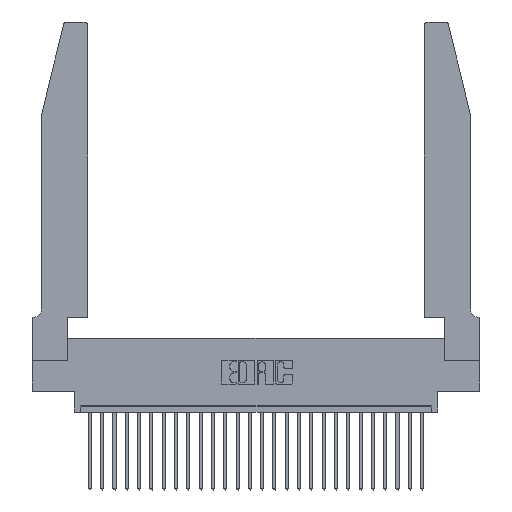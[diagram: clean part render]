
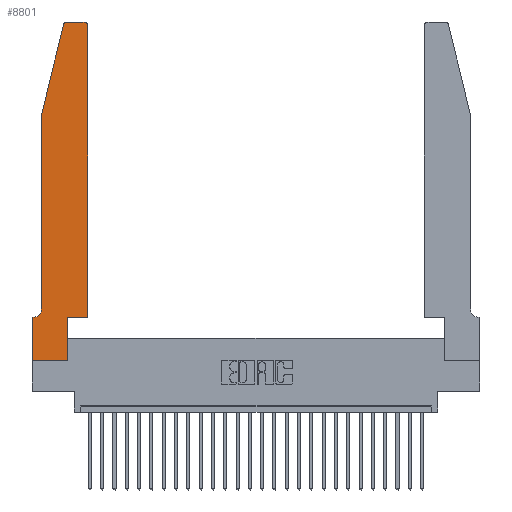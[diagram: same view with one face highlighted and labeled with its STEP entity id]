
A CAD part, top view. The second image highlights one B-rep face of the part: STEP entity #8801.
In plain terms, the highlighted planar face has unit normal (0, 0, 1).
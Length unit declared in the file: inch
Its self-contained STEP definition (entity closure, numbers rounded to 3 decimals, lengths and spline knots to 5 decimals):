
#81 = VERTEX_POINT ( 'NONE', #21621 ) ;
#365 = ORIENTED_EDGE ( 'NONE', *, *, #10234, .T. ) ;
#627 = DIRECTION ( 'NONE',  ( 0., 0., 1. ) ) ;
#1090 = CARTESIAN_POINT ( 'NONE',  ( 0.4205, 2.75, 0.37 ) ) ;
#1099 = EDGE_CURVE ( 'NONE', #7699, #81, #10489, .T. ) ;
#1174 = VECTOR ( 'NONE', #8056, 39.37008 ) ;
#1873 = ORIENTED_EDGE ( 'NONE', *, *, #8863, .T. ) ;
#1979 = DIRECTION ( 'NONE',  ( -0.239, -0.971, 0. ) ) ;
#1986 = CIRCLE ( 'NONE', #18469, 0.03 ) ;
#2052 = CARTESIAN_POINT ( 'NONE',  ( 0., 0., 0.37 ) ) ;
#2058 = CARTESIAN_POINT ( 'NONE',  ( 0.0055, 0.42, 0.37 ) ) ;
#2445 = DIRECTION ( 'NONE',  ( 0., 0., 1. ) ) ;
#2933 = VERTEX_POINT ( 'NONE', #11537 ) ;
#3525 = DIRECTION ( 'NONE',  ( 1., 0., 0. ) ) ;
#3852 = EDGE_CURVE ( 'NONE', #22568, #19547, #4517, .T. ) ;
#3882 = VECTOR ( 'NONE', #3525, 39.37008 ) ;
#4231 = LINE ( 'NONE', #16467, #1174 ) ;
#4517 = LINE ( 'NONE', #2052, #8224 ) ;
#4725 = LINE ( 'NONE', #13788, #12792 ) ;
#5805 = CARTESIAN_POINT ( 'NONE',  ( 0., 0.35, 0.37 ) ) ;
#6285 = EDGE_CURVE ( 'NONE', #2933, #8730, #16114, .T. ) ;
#6507 = DIRECTION ( 'NONE',  ( 0., 1., 0. ) ) ;
#6739 = CARTESIAN_POINT ( 'NONE',  ( 0.2865, 0.35, 0.37 ) ) ;
#7037 = ORIENTED_EDGE ( 'NONE', *, *, #1099, .T. ) ;
#7048 = CARTESIAN_POINT ( 'NONE',  ( 0.25487, 2.72718, 0.37 ) ) ;
#7078 = ORIENTED_EDGE ( 'NONE', *, *, #12783, .T. ) ;
#7085 = VERTEX_POINT ( 'NONE', #16417 ) ;
#7314 = EDGE_CURVE ( 'NONE', #25011, #2933, #10383, .T. ) ;
#7699 = VERTEX_POINT ( 'NONE', #15343 ) ;
#8056 = DIRECTION ( 'NONE',  ( 0., -1., 0. ) ) ;
#8224 = VECTOR ( 'NONE', #12958, 39.37008 ) ;
#8242 = DIRECTION ( 'NONE',  ( 0., 1., 0. ) ) ;
#8587 = PLANE ( 'NONE',  #19742 ) ;
#8730 = VERTEX_POINT ( 'NONE', #18308 ) ;
#8801 = ADVANCED_FACE ( 'NONE', ( #24024 ), #8587, .T. ) ;
#8846 = CARTESIAN_POINT ( 'NONE',  ( 0.4205, 2.72, 0.37 ) ) ;
#8863 = EDGE_CURVE ( 'NONE', #19478, #7699, #4231, .T. ) ;
#8915 = ORIENTED_EDGE ( 'NONE', *, *, #7314, .T. ) ;
#9138 = VECTOR ( 'NONE', #1979, 39.37008 ) ;
#9462 = CARTESIAN_POINT ( 'NONE',  ( 0.4505, 0.35, 0.37 ) ) ;
#10234 = EDGE_CURVE ( 'NONE', #19547, #7085, #21976, .T. ) ;
#10359 = LINE ( 'NONE', #15469, #25104 ) ;
#10383 = LINE ( 'NONE', #9462, #20718 ) ;
#10391 = ORIENTED_EDGE ( 'NONE', *, *, #14612, .T. ) ;
#10489 = CIRCLE ( 'NONE', #17166, 0.07 ) ;
#10871 = VERTEX_POINT ( 'NONE', #11528 ) ;
#11095 = DIRECTION ( 'NONE',  ( 1., 0., 0. ) ) ;
#11096 = DIRECTION ( 'NONE',  ( 1., 0., 0. ) ) ;
#11528 = CARTESIAN_POINT ( 'NONE',  ( 0.284, 2.75, 0.37 ) ) ;
#11537 = CARTESIAN_POINT ( 'NONE',  ( 0.4505, 0.35, 0.37 ) ) ;
#11760 = ORIENTED_EDGE ( 'NONE', *, *, #15608, .T. ) ;
#11919 = DIRECTION ( 'NONE',  ( 1., 0., 0. ) ) ;
#12475 = VERTEX_POINT ( 'NONE', #1090 ) ;
#12671 = CARTESIAN_POINT ( 'NONE',  ( 0., 0.35, 0.37 ) ) ;
#12770 = VECTOR ( 'NONE', #6507, 39.37008 ) ;
#12783 = EDGE_CURVE ( 'NONE', #81, #22568, #4725, .T. ) ;
#12792 = VECTOR ( 'NONE', #14840, 39.37008 ) ;
#12958 = DIRECTION ( 'NONE',  ( 0., -1., 0. ) ) ;
#13049 = DIRECTION ( 'NONE',  ( -1., 0., 0. ) ) ;
#13065 = CARTESIAN_POINT ( 'NONE',  ( 0.0755, 2., 0.37 ) ) ;
#13522 = CARTESIAN_POINT ( 'NONE',  ( 0.284, 2.72, 0.37 ) ) ;
#13788 = CARTESIAN_POINT ( 'NONE',  ( 0.0755, 0.35, 0.37 ) ) ;
#14048 = CARTESIAN_POINT ( 'NONE',  ( 0., 0., 0.37 ) ) ;
#14078 = VECTOR ( 'NONE', #8242, 39.37008 ) ;
#14612 = EDGE_CURVE ( 'NONE', #12475, #10871, #10359, .T. ) ;
#14840 = DIRECTION ( 'NONE',  ( -1., 0., 0. ) ) ;
#15343 = CARTESIAN_POINT ( 'NONE',  ( 0.0755, 0.42, 0.37 ) ) ;
#15469 = CARTESIAN_POINT ( 'NONE',  ( 0.2605, 2.75, 0.37 ) ) ;
#15608 = EDGE_CURVE ( 'NONE', #10871, #26578, #1986, .T. ) ;
#15886 = EDGE_CURVE ( 'NONE', #7085, #25011, #26161, .T. ) ;
#16114 = LINE ( 'NONE', #23655, #12770 ) ;
#16274 = ORIENTED_EDGE ( 'NONE', *, *, #24451, .T. ) ;
#16417 = CARTESIAN_POINT ( 'NONE',  ( 0.2865, 0., 0.37 ) ) ;
#16467 = CARTESIAN_POINT ( 'NONE',  ( 0.0755, 2., 0.37 ) ) ;
#16665 = DIRECTION ( 'NONE',  ( 1., 0., 0. ) ) ;
#17166 = AXIS2_PLACEMENT_3D ( 'NONE', #2058, #25899, #13049 ) ;
#17295 = DIRECTION ( 'NONE',  ( 0., 0., 1. ) ) ;
#18308 = CARTESIAN_POINT ( 'NONE',  ( 0.4505, 2.72, 0.37 ) ) ;
#18469 = AXIS2_PLACEMENT_3D ( 'NONE', #13522, #627, #11919 ) ;
#19478 = VERTEX_POINT ( 'NONE', #23539 ) ;
#19501 = ORIENTED_EDGE ( 'NONE', *, *, #6285, .T. ) ;
#19547 = VERTEX_POINT ( 'NONE', #25784 ) ;
#19742 = AXIS2_PLACEMENT_3D ( 'NONE', #5805, #17295, #11095 ) ;
#19944 = ORIENTED_EDGE ( 'NONE', *, *, #3852, .T. ) ;
#20227 = AXIS2_PLACEMENT_3D ( 'NONE', #8846, #2445, #11096 ) ;
#20520 = LINE ( 'NONE', #13065, #9138 ) ;
#20718 = VECTOR ( 'NONE', #16665, 39.37008 ) ;
#21520 = CIRCLE ( 'NONE', #20227, 0.03 ) ;
#21621 = CARTESIAN_POINT ( 'NONE',  ( 0.0055, 0.35, 0.37 ) ) ;
#21976 = LINE ( 'NONE', #14048, #3882 ) ;
#22046 = EDGE_CURVE ( 'NONE', #26578, #19478, #20520, .T. ) ;
#22463 = DIRECTION ( 'NONE',  ( -1., 0., 0. ) ) ;
#22568 = VERTEX_POINT ( 'NONE', #12671 ) ;
#23327 = ORIENTED_EDGE ( 'NONE', *, *, #22046, .T. ) ;
#23539 = CARTESIAN_POINT ( 'NONE',  ( 0.0755, 2., 0.37 ) ) ;
#23655 = CARTESIAN_POINT ( 'NONE',  ( 0.4505, 0.35, 0.37 ) ) ;
#23706 = ORIENTED_EDGE ( 'NONE', *, *, #15886, .T. ) ;
#24024 = FACE_OUTER_BOUND ( 'NONE', #26469, .T. ) ;
#24451 = EDGE_CURVE ( 'NONE', #8730, #12475, #21520, .T. ) ;
#25011 = VERTEX_POINT ( 'NONE', #6739 ) ;
#25104 = VECTOR ( 'NONE', #22463, 39.37008 ) ;
#25784 = CARTESIAN_POINT ( 'NONE',  ( 0., 0., 0.37 ) ) ;
#25899 = DIRECTION ( 'NONE',  ( 0., 0., -1. ) ) ;
#26161 = LINE ( 'NONE', #27374, #14078 ) ;
#26469 = EDGE_LOOP ( 'NONE', ( #10391, #11760, #23327, #1873, #7037, #7078, #19944, #365, #23706, #8915, #19501, #16274 ) ) ;
#26578 = VERTEX_POINT ( 'NONE', #7048 ) ;
#27374 = CARTESIAN_POINT ( 'NONE',  ( 0.2865, 0.35, 0.37 ) ) ;
